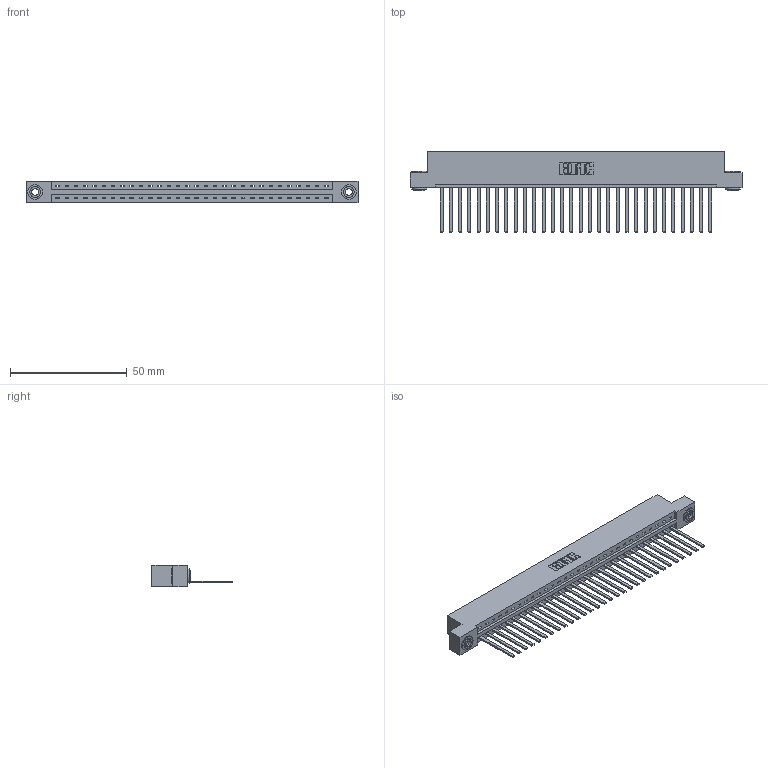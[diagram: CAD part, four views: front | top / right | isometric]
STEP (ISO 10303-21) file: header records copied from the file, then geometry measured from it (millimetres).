
FILE_DESCRIPTION (( 'STEP AP203' ), '1' );
FILE_NAME ('337-030-544-103.STEP', '2018-08-07T01:37:07', ( '' ), ( '' ), 'SwSTEP 2.0', 'SolidWorks 2016', '' );
FILE_SCHEMA (( 'CONFIG_CONTROL_DESIGN' ));
Length unit declared in the file: inch
Products named in the file (4): 345-292-001_345-293-144; 345-250-002_345-250-002-102; 337-030-544-103; 337 Part_Flush Mounting Lugs - 0.156 Dia-TH
Assembly tree (33 placements, depth 2):
  337-030-544-103
    337 Part_Flush Mounting Lugs - 0.156 Dia-TH
    345-292-001_345-293-144  x30
    345-250-002_345-250-002-102  x2
Bounding box: 141.88 x 34.3 x 9.4 mm (x, y, z)
Volume: 14963.2 mm3; surface area: 16771.3 mm2
Topology: 33 solids, 33 shells, 1832 faces, 5487 edges, 3614 vertices
Faces by surface type: plane 1340, cylinder 484, cone 8
Entity records: 24318 total; most frequent: CARTESIAN_POINT 4211, ORIENTED_EDGE 4170, DIRECTION 3599, EDGE_CURVE 2085, LINE 1937, VECTOR 1937, VERTEX_POINT 1386, AXIS2_PLACEMENT_3D 831
